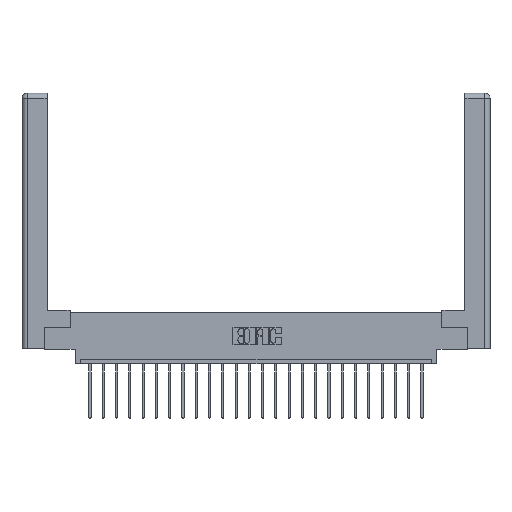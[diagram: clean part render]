
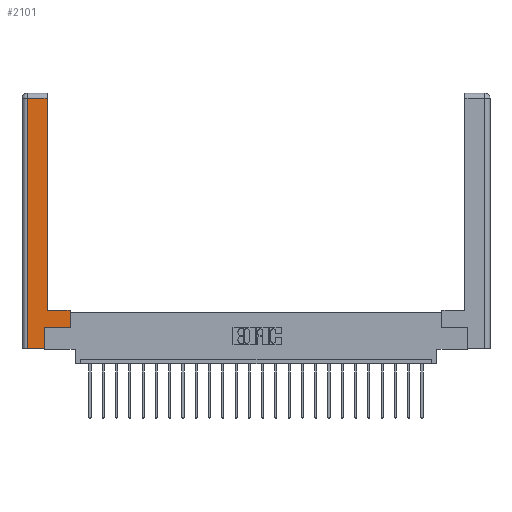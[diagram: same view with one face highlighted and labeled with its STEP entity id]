
A CAD part, top view. The second image highlights one B-rep face of the part: STEP entity #2101.
In plain terms, the highlighted planar face has unit normal (0, 0, 1).
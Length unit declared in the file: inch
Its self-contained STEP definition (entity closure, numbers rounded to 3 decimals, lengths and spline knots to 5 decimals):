
#130 = EDGE_CURVE ( 'NONE', #12709, #15865, #23824, .T. ) ;
#210 = AXIS2_PLACEMENT_3D ( 'NONE', #13750, #2598, #4493 ) ;
#458 = DIRECTION ( 'NONE',  ( 1., 0., 0. ) ) ;
#487 = LINE ( 'NONE', #11660, #19165 ) ;
#744 = PLANE ( 'NONE',  #210 ) ;
#789 = CARTESIAN_POINT ( 'NONE',  ( 0.295, 0.45, 0. ) ) ;
#1459 = VERTEX_POINT ( 'NONE', #11511 ) ;
#2101 = ADVANCED_FACE ( 'NONE', ( #20796 ), #744, .F. ) ;
#2379 = DIRECTION ( 'NONE',  ( 0., 1., 0. ) ) ;
#2488 = CARTESIAN_POINT ( 'NONE',  ( 0.565, 0.45, 0. ) ) ;
#2598 = DIRECTION ( 'NONE',  ( 0., 0., -1. ) ) ;
#2736 = EDGE_CURVE ( 'NONE', #10890, #12709, #15741, .T. ) ;
#3038 = DIRECTION ( 'NONE',  ( 0., 1., 0. ) ) ;
#3045 = ORIENTED_EDGE ( 'NONE', *, *, #130, .T. ) ;
#3056 = CARTESIAN_POINT ( 'NONE',  ( 0.0615, 2.94, 0. ) ) ;
#3323 = LINE ( 'NONE', #9380, #10306 ) ;
#3380 = CARTESIAN_POINT ( 'NONE',  ( 0.265, 0.245, 0. ) ) ;
#4493 = DIRECTION ( 'NONE',  ( -1., 0., 0. ) ) ;
#4815 = LINE ( 'NONE', #21576, #12690 ) ;
#5549 = LINE ( 'NONE', #3056, #14279 ) ;
#5592 = VERTEX_POINT ( 'NONE', #12411 ) ;
#6001 = EDGE_CURVE ( 'NONE', #22422, #9702, #5549, .T. ) ;
#6132 = VECTOR ( 'NONE', #3038, 39.37008 ) ;
#6602 = CARTESIAN_POINT ( 'NONE',  ( 0.295, 2.94, 0. ) ) ;
#6874 = EDGE_CURVE ( 'NONE', #17974, #10890, #3323, .T. ) ;
#7319 = VECTOR ( 'NONE', #8496, 39.37008 ) ;
#8023 = ORIENTED_EDGE ( 'NONE', *, *, #13836, .T. ) ;
#8496 = DIRECTION ( 'NONE',  ( 0., 1., 0. ) ) ;
#8913 = CARTESIAN_POINT ( 'NONE',  ( 0.565, 0.245, 0. ) ) ;
#9229 = LINE ( 'NONE', #15574, #22990 ) ;
#9331 = ORIENTED_EDGE ( 'NONE', *, *, #19221, .T. ) ;
#9380 = CARTESIAN_POINT ( 'NONE',  ( 0.565, 0.245, 0. ) ) ;
#9384 = ORIENTED_EDGE ( 'NONE', *, *, #2736, .T. ) ;
#9702 = VERTEX_POINT ( 'NONE', #16359 ) ;
#9865 = EDGE_LOOP ( 'NONE', ( #14164, #21247, #16474, #9331, #8023, #21825, #9384, #3045 ) ) ;
#10182 = DIRECTION ( 'NONE',  ( -1., 0., 0. ) ) ;
#10295 = CARTESIAN_POINT ( 'NONE',  ( 0.565, 0.45, 0. ) ) ;
#10306 = VECTOR ( 'NONE', #11243, 39.37008 ) ;
#10366 = VECTOR ( 'NONE', #10182, 39.37008 ) ;
#10628 = DIRECTION ( 'NONE',  ( 0., -1., 0. ) ) ;
#10845 = EDGE_CURVE ( 'NONE', #15865, #22422, #21933, .T. ) ;
#10890 = VERTEX_POINT ( 'NONE', #8913 ) ;
#11243 = DIRECTION ( 'NONE',  ( 1., 0., 0. ) ) ;
#11511 = CARTESIAN_POINT ( 'NONE',  ( 0.0615, 0., 0. ) ) ;
#11660 = CARTESIAN_POINT ( 'NONE',  ( 0.265, 0.245, 0. ) ) ;
#12411 = CARTESIAN_POINT ( 'NONE',  ( 0.265, 0., 0. ) ) ;
#12690 = VECTOR ( 'NONE', #10628, 39.37008 ) ;
#12709 = VERTEX_POINT ( 'NONE', #2488 ) ;
#13750 = CARTESIAN_POINT ( 'NONE',  ( 0., 0., 0. ) ) ;
#13836 = EDGE_CURVE ( 'NONE', #5592, #17974, #487, .T. ) ;
#14111 = CARTESIAN_POINT ( 'NONE',  ( 0.295, 3., 0. ) ) ;
#14164 = ORIENTED_EDGE ( 'NONE', *, *, #10845, .T. ) ;
#14279 = VECTOR ( 'NONE', #14362, 39.37008 ) ;
#14362 = DIRECTION ( 'NONE',  ( -1., 0., 0. ) ) ;
#14967 = EDGE_CURVE ( 'NONE', #9702, #1459, #4815, .T. ) ;
#15574 = CARTESIAN_POINT ( 'NONE',  ( 0.265, 0., 0. ) ) ;
#15741 = LINE ( 'NONE', #10295, #7319 ) ;
#15865 = VERTEX_POINT ( 'NONE', #789 ) ;
#16359 = CARTESIAN_POINT ( 'NONE',  ( 0.0615, 2.94, 0. ) ) ;
#16474 = ORIENTED_EDGE ( 'NONE', *, *, #14967, .T. ) ;
#17768 = CARTESIAN_POINT ( 'NONE',  ( 0.295, 0.45, 0. ) ) ;
#17974 = VERTEX_POINT ( 'NONE', #3380 ) ;
#19165 = VECTOR ( 'NONE', #2379, 39.37008 ) ;
#19221 = EDGE_CURVE ( 'NONE', #1459, #5592, #9229, .T. ) ;
#20796 = FACE_OUTER_BOUND ( 'NONE', #9865, .T. ) ;
#21247 = ORIENTED_EDGE ( 'NONE', *, *, #6001, .T. ) ;
#21576 = CARTESIAN_POINT ( 'NONE',  ( 0.0615, 0., 0. ) ) ;
#21825 = ORIENTED_EDGE ( 'NONE', *, *, #6874, .T. ) ;
#21933 = LINE ( 'NONE', #14111, #6132 ) ;
#22422 = VERTEX_POINT ( 'NONE', #6602 ) ;
#22990 = VECTOR ( 'NONE', #458, 39.37008 ) ;
#23824 = LINE ( 'NONE', #17768, #10366 ) ;
